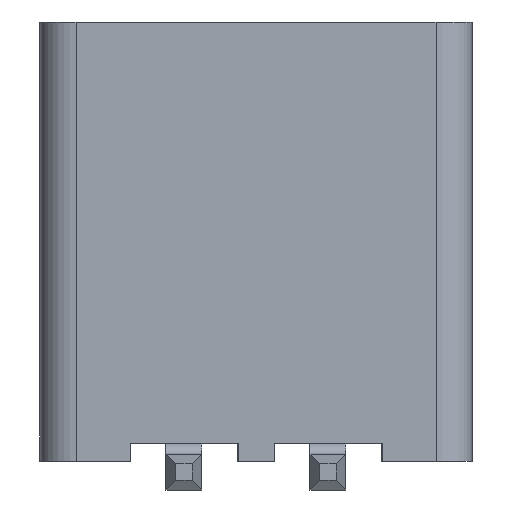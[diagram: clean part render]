
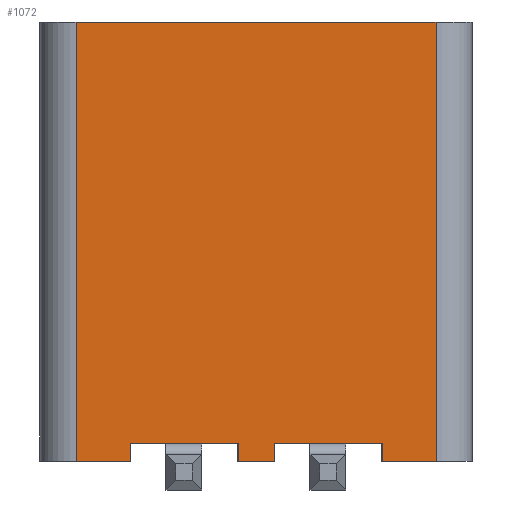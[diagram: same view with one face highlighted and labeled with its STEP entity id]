
A CAD part, front view. The second image highlights one B-rep face of the part: STEP entity #1072.
In plain terms, the highlighted planar face has unit normal (0, -1, 0).
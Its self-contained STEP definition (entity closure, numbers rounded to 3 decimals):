
#14 = VERTEX_POINT ( 'NONE', #304 ) ;
#20 = EDGE_CURVE ( 'NONE', #751, #2041, #1148, .T. ) ;
#42 = CARTESIAN_POINT ( 'NONE',  ( 1.25, -2.7, 0. ) ) ;
#72 = VECTOR ( 'NONE', #1776, 1000. ) ;
#128 = ORIENTED_EDGE ( 'NONE', *, *, #677, .T. ) ;
#137 = DIRECTION ( 'NONE',  ( 0., 0., -1. ) ) ;
#197 = EDGE_CURVE ( 'NONE', #1345, #1150, #1614, .T. ) ;
#221 = DIRECTION ( 'NONE',  ( 0., 0., -1. ) ) ;
#239 = ORIENTED_EDGE ( 'NONE', *, *, #1768, .T. ) ;
#283 = LINE ( 'NONE', #1967, #72 ) ;
#304 = CARTESIAN_POINT ( 'NONE',  ( 0.75, -2.7, 0.25 ) ) ;
#359 = CARTESIAN_POINT ( 'NONE',  ( -1.5, -2.7, 0. ) ) ;
#376 = EDGE_LOOP ( 'NONE', ( #1436, #1939, #620, #1618, #2569, #1710, #239, #1047, #1449, #2116, #128, #1812 ) ) ;
#385 = EDGE_CURVE ( 'NONE', #1022, #14, #1857, .T. ) ;
#404 = CARTESIAN_POINT ( 'NONE',  ( 2.75, -2.7, 0.25 ) ) ;
#423 = VECTOR ( 'NONE', #2647, 1000. ) ;
#431 = DIRECTION ( 'NONE',  ( 0., -1., 0. ) ) ;
#499 = EDGE_CURVE ( 'NONE', #1546, #1345, #1645, .T. ) ;
#507 = DIRECTION ( 'NONE',  ( 0., 0., 1. ) ) ;
#508 = VERTEX_POINT ( 'NONE', #2364 ) ;
#554 = EDGE_CURVE ( 'NONE', #14, #508, #2543, .T. ) ;
#564 = VECTOR ( 'NONE', #2239, 1000. ) ;
#604 = VECTOR ( 'NONE', #823, 1000. ) ;
#620 = ORIENTED_EDGE ( 'NONE', *, *, #499, .T. ) ;
#648 = CARTESIAN_POINT ( 'NONE',  ( 3.5, -2.7, 6.1 ) ) ;
#677 = EDGE_CURVE ( 'NONE', #1262, #751, #1180, .T. ) ;
#751 = VERTEX_POINT ( 'NONE', #949 ) ;
#780 = CARTESIAN_POINT ( 'NONE',  ( 2.75, -2.7, 0. ) ) ;
#799 = LINE ( 'NONE', #1198, #1964 ) ;
#823 = DIRECTION ( 'NONE',  ( -1., 0., 0. ) ) ;
#848 = VERTEX_POINT ( 'NONE', #780 ) ;
#852 = VECTOR ( 'NONE', #2113, 1000. ) ;
#875 = LINE ( 'NONE', #2719, #604 ) ;
#911 = LINE ( 'NONE', #2177, #1672 ) ;
#918 = DIRECTION ( 'NONE',  ( 0., 0., 1. ) ) ;
#928 = CARTESIAN_POINT ( 'NONE',  ( 2.75, -2.7, 0.25 ) ) ;
#944 = CARTESIAN_POINT ( 'NONE',  ( 2.75, -2.7, 0.25 ) ) ;
#949 = CARTESIAN_POINT ( 'NONE',  ( 1.25, -2.7, 0.25 ) ) ;
#1010 = CARTESIAN_POINT ( 'NONE',  ( -0.75, -2.7, 0.25 ) ) ;
#1022 = VERTEX_POINT ( 'NONE', #1010 ) ;
#1034 = LINE ( 'NONE', #404, #2296 ) ;
#1047 = ORIENTED_EDGE ( 'NONE', *, *, #385, .T. ) ;
#1048 = VECTOR ( 'NONE', #1422, 1000. ) ;
#1072 = ADVANCED_FACE ( 'NONE', ( #2082 ), #2709, .T. ) ;
#1096 = EDGE_CURVE ( 'NONE', #2041, #848, #1034, .T. ) ;
#1148 = LINE ( 'NONE', #944, #423 ) ;
#1150 = VERTEX_POINT ( 'NONE', #1469 ) ;
#1180 = LINE ( 'NONE', #2183, #1512 ) ;
#1198 = CARTESIAN_POINT ( 'NONE',  ( -1.5, -2.7, 6.1 ) ) ;
#1262 = VERTEX_POINT ( 'NONE', #42 ) ;
#1345 = VERTEX_POINT ( 'NONE', #2242 ) ;
#1422 = DIRECTION ( 'NONE',  ( 1., 0., 0. ) ) ;
#1436 = ORIENTED_EDGE ( 'NONE', *, *, #1096, .T. ) ;
#1449 = ORIENTED_EDGE ( 'NONE', *, *, #554, .T. ) ;
#1469 = CARTESIAN_POINT ( 'NONE',  ( -1.5, -2.7, 6.1 ) ) ;
#1512 = VECTOR ( 'NONE', #1996, 1000. ) ;
#1546 = VERTEX_POINT ( 'NONE', #2581 ) ;
#1614 = LINE ( 'NONE', #1851, #564 ) ;
#1618 = ORIENTED_EDGE ( 'NONE', *, *, #197, .T. ) ;
#1645 = LINE ( 'NONE', #648, #2024 ) ;
#1661 = VECTOR ( 'NONE', #2592, 1000. ) ;
#1672 = VECTOR ( 'NONE', #507, 1000. ) ;
#1710 = ORIENTED_EDGE ( 'NONE', *, *, #2426, .F. ) ;
#1722 = AXIS2_PLACEMENT_3D ( 'NONE', #2310, #431, #2125 ) ;
#1760 = LINE ( 'NONE', #2564, #1661 ) ;
#1768 = EDGE_CURVE ( 'NONE', #2435, #1022, #911, .T. ) ;
#1776 = DIRECTION ( 'NONE',  ( -1., 0., 0. ) ) ;
#1812 = ORIENTED_EDGE ( 'NONE', *, *, #20, .T. ) ;
#1851 = CARTESIAN_POINT ( 'NONE',  ( 4., -2.7, 6.1 ) ) ;
#1857 = LINE ( 'NONE', #2716, #1048 ) ;
#1883 = EDGE_CURVE ( 'NONE', #1546, #848, #1760, .T. ) ;
#1932 = CARTESIAN_POINT ( 'NONE',  ( 0.75, -2.7, 0.25 ) ) ;
#1939 = ORIENTED_EDGE ( 'NONE', *, *, #1883, .F. ) ;
#1964 = VECTOR ( 'NONE', #137, 1000. ) ;
#1967 = CARTESIAN_POINT ( 'NONE',  ( 4., -2.7, 0. ) ) ;
#1996 = DIRECTION ( 'NONE',  ( 0., 0., 1. ) ) ;
#2024 = VECTOR ( 'NONE', #918, 1000. ) ;
#2041 = VERTEX_POINT ( 'NONE', #928 ) ;
#2059 = EDGE_CURVE ( 'NONE', #1262, #508, #283, .T. ) ;
#2082 = FACE_OUTER_BOUND ( 'NONE', #376, .T. ) ;
#2113 = DIRECTION ( 'NONE',  ( 0., 0., -1. ) ) ;
#2116 = ORIENTED_EDGE ( 'NONE', *, *, #2059, .F. ) ;
#2125 = DIRECTION ( 'NONE',  ( 0., 0., 1. ) ) ;
#2158 = CARTESIAN_POINT ( 'NONE',  ( -0.75, -2.7, 0. ) ) ;
#2177 = CARTESIAN_POINT ( 'NONE',  ( -0.75, -2.7, 0.25 ) ) ;
#2183 = CARTESIAN_POINT ( 'NONE',  ( 1.25, -2.7, 0.25 ) ) ;
#2236 = VERTEX_POINT ( 'NONE', #359 ) ;
#2239 = DIRECTION ( 'NONE',  ( -1., 0., 0. ) ) ;
#2242 = CARTESIAN_POINT ( 'NONE',  ( 3.5, -2.7, 6.1 ) ) ;
#2296 = VECTOR ( 'NONE', #221, 1000. ) ;
#2310 = CARTESIAN_POINT ( 'NONE',  ( 4., -2.7, 6.1 ) ) ;
#2364 = CARTESIAN_POINT ( 'NONE',  ( 0.75, -2.7, 0. ) ) ;
#2426 = EDGE_CURVE ( 'NONE', #2435, #2236, #875, .T. ) ;
#2435 = VERTEX_POINT ( 'NONE', #2158 ) ;
#2543 = LINE ( 'NONE', #1932, #852 ) ;
#2564 = CARTESIAN_POINT ( 'NONE',  ( 4., -2.7, 0. ) ) ;
#2569 = ORIENTED_EDGE ( 'NONE', *, *, #2589, .T. ) ;
#2581 = CARTESIAN_POINT ( 'NONE',  ( 3.5, -2.7, 0. ) ) ;
#2589 = EDGE_CURVE ( 'NONE', #1150, #2236, #799, .T. ) ;
#2592 = DIRECTION ( 'NONE',  ( -1., 0., 0. ) ) ;
#2647 = DIRECTION ( 'NONE',  ( 1., 0., 0. ) ) ;
#2709 = PLANE ( 'NONE',  #1722 ) ;
#2716 = CARTESIAN_POINT ( 'NONE',  ( 0.75, -2.7, 0.25 ) ) ;
#2719 = CARTESIAN_POINT ( 'NONE',  ( 4., -2.7, 0. ) ) ;
